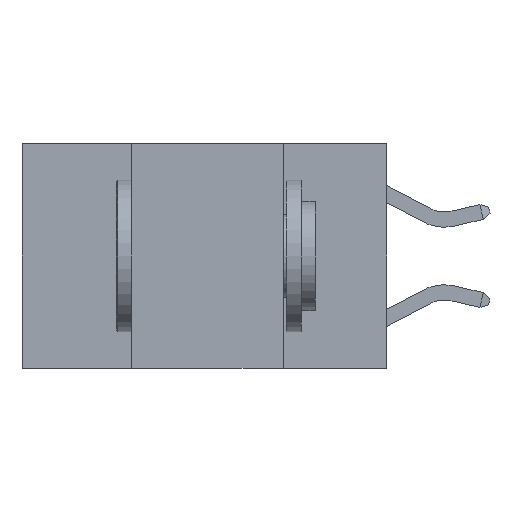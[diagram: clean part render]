
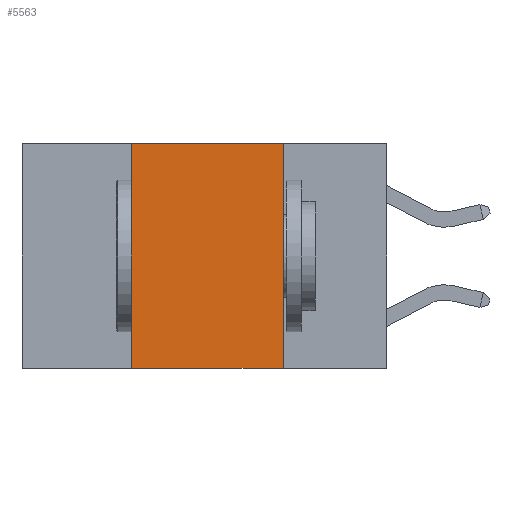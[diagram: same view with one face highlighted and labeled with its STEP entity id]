
A CAD part, left-side view. The second image highlights one B-rep face of the part: STEP entity #5563.
In plain terms, the highlighted planar face has unit normal (-1, 0, 0).
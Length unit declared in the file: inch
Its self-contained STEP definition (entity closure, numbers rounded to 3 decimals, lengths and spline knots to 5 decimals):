
#126 = CARTESIAN_POINT ( 'NONE',  ( 0., 0.6, -0.37 ) ) ;
#205 = VERTEX_POINT ( 'NONE', #4814 ) ;
#305 = ORIENTED_EDGE ( 'NONE', *, *, #9231, .F. ) ;
#409 = EDGE_CURVE ( 'NONE', #8346, #205, #3449, .T. ) ;
#484 = VECTOR ( 'NONE', #7415, 39.37008 ) ;
#947 = DIRECTION ( 'NONE',  ( 0., -1., 0. ) ) ;
#1003 = LINE ( 'NONE', #126, #6726 ) ;
#1825 = VERTEX_POINT ( 'NONE', #7003 ) ;
#2273 = ORIENTED_EDGE ( 'NONE', *, *, #409, .F. ) ;
#2481 = DIRECTION ( 'NONE',  ( 1., 0., 0. ) ) ;
#2522 = ORIENTED_EDGE ( 'NONE', *, *, #7666, .T. ) ;
#2569 = AXIS2_PLACEMENT_3D ( 'NONE', #8725, #2481, #7507 ) ;
#2668 = CARTESIAN_POINT ( 'NONE',  ( 0., 0.42, 0. ) ) ;
#3227 = VECTOR ( 'NONE', #8533, 39.37008 ) ;
#3388 = DIRECTION ( 'NONE',  ( 0., 0., 1. ) ) ;
#3449 = LINE ( 'NONE', #8998, #3227 ) ;
#4152 = VERTEX_POINT ( 'NONE', #8084 ) ;
#4167 = ORIENTED_EDGE ( 'NONE', *, *, #6705, .F. ) ;
#4814 = CARTESIAN_POINT ( 'NONE',  ( 0., 0.17, -0.37 ) ) ;
#5520 = LINE ( 'NONE', #2668, #8890 ) ;
#5563 = ADVANCED_FACE ( 'NONE', ( #6661 ), #6806, .F. ) ;
#6661 = FACE_OUTER_BOUND ( 'NONE', #8122, .T. ) ;
#6705 = EDGE_CURVE ( 'NONE', #1825, #8346, #8314, .T. ) ;
#6719 = CARTESIAN_POINT ( 'NONE',  ( 0., 0.6, 0. ) ) ;
#6726 = VECTOR ( 'NONE', #947, 39.37008 ) ;
#6806 = PLANE ( 'NONE',  #2569 ) ;
#6897 = CARTESIAN_POINT ( 'NONE',  ( 0., 0.17, 0. ) ) ;
#7003 = CARTESIAN_POINT ( 'NONE',  ( 0., 0.42, 0. ) ) ;
#7415 = DIRECTION ( 'NONE',  ( 0., -1., 0. ) ) ;
#7507 = DIRECTION ( 'NONE',  ( 0., 0., -1. ) ) ;
#7666 = EDGE_CURVE ( 'NONE', #4152, #205, #1003, .T. ) ;
#8084 = CARTESIAN_POINT ( 'NONE',  ( 0., 0.42, -0.37 ) ) ;
#8122 = EDGE_LOOP ( 'NONE', ( #2273, #4167, #305, #2522 ) ) ;
#8314 = LINE ( 'NONE', #6719, #484 ) ;
#8346 = VERTEX_POINT ( 'NONE', #6897 ) ;
#8533 = DIRECTION ( 'NONE',  ( 0., 0., -1. ) ) ;
#8725 = CARTESIAN_POINT ( 'NONE',  ( 0., 0.6, 0. ) ) ;
#8890 = VECTOR ( 'NONE', #3388, 39.37008 ) ;
#8998 = CARTESIAN_POINT ( 'NONE',  ( 0., 0.17, 0. ) ) ;
#9231 = EDGE_CURVE ( 'NONE', #4152, #1825, #5520, .T. ) ;
